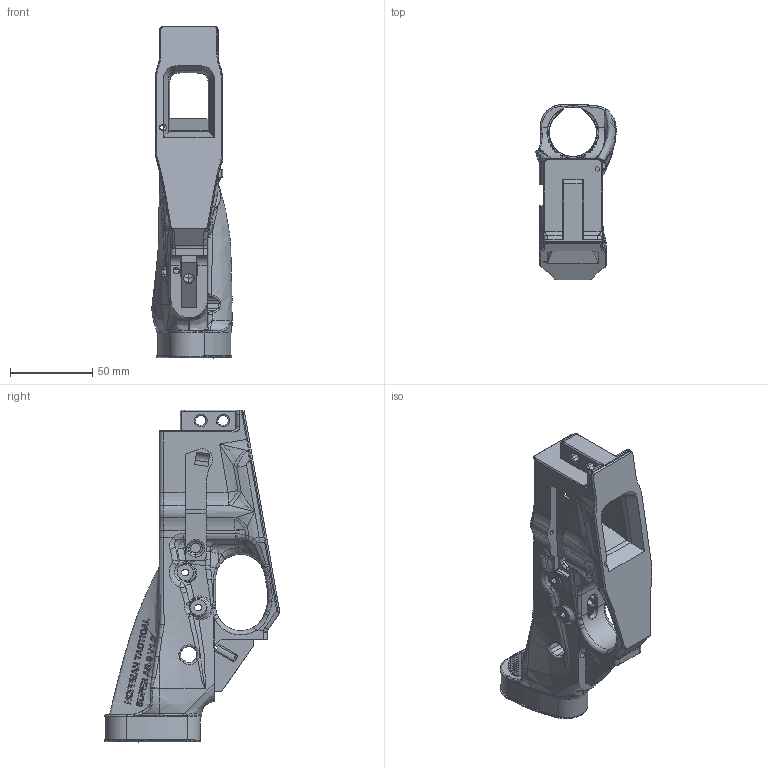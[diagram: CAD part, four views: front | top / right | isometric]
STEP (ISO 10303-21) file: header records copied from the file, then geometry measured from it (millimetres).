
FILE_DESCRIPTION (( 'STEP AP203' ), '1' );
FILE_NAME ('AR-9 SL NS V1.2.STEP', '2022-07-31T18:53:23', ( '' ), ( '' ), 'SwSTEP 2.0', 'SolidWorks 2021', '' );
FILE_SCHEMA (( 'CONFIG_CONTROL_DESIGN' ));
Products named in the file (1): AR-9 SL NS V1.2
Bounding box: 48.72 x 106.75 x 201.55 mm (x, y, z)
Volume: 214964.4 mm3; surface area: 65309.7 mm2
Topology: 1 solids, 1 shells, 1806 faces, 4832 edges, 3061 vertices
Faces by surface type: bspline 1049, plane 329, cylinder 297, torus 79, cone 37, sphere 15
Entity records: 246625 total; most frequent: CARTESIAN_POINT 210552, ORIENTED_EDGE 9590, EDGE_CURVE 4795, DIRECTION 4300, VERTEX_POINT 3061, B_SPLINE_CURVE_WITH_KNOTS 2497, EDGE_LOOP 1922, ADVANCED_FACE 1806
